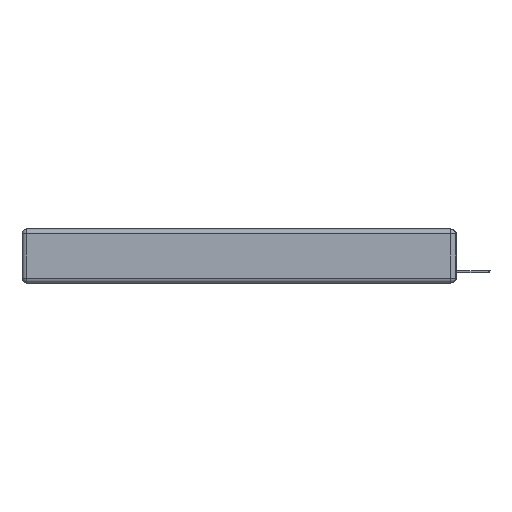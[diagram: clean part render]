
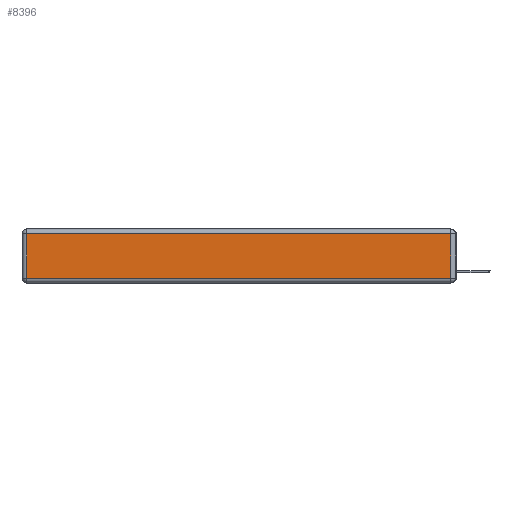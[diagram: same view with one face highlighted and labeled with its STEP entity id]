
A CAD part, left-side view. The second image highlights one B-rep face of the part: STEP entity #8396.
In plain terms, the highlighted planar face has unit normal (-1, 0, 0).
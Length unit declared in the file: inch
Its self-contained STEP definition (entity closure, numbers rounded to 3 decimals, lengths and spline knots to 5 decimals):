
#834 = DIRECTION ( 'NONE',  ( 0., -1., 0. ) ) ;
#1921 = CARTESIAN_POINT ( 'NONE',  ( 0., 0.03, -0.313 ) ) ;
#1926 = VECTOR ( 'NONE', #834, 39.37008 ) ;
#2035 = CARTESIAN_POINT ( 'NONE',  ( 0., 0.03, -0.03 ) ) ;
#2596 = DIRECTION ( 'NONE',  ( -1., 0., 0. ) ) ;
#2621 = ORIENTED_EDGE ( 'NONE', *, *, #5702, .T. ) ;
#3609 = DIRECTION ( 'NONE',  ( 0., 0., 1. ) ) ;
#3985 = VECTOR ( 'NONE', #3609, 39.37008 ) ;
#4456 = LINE ( 'NONE', #26668, #16913 ) ;
#4684 = VERTEX_POINT ( 'NONE', #1921 ) ;
#5519 = VERTEX_POINT ( 'NONE', #24535 ) ;
#5702 = EDGE_CURVE ( 'NONE', #12325, #5519, #23433, .T. ) ;
#5783 = CARTESIAN_POINT ( 'NONE',  ( 0., 0.03, -0.343 ) ) ;
#6226 = DIRECTION ( 'NONE',  ( 0., 1., 0. ) ) ;
#6481 = CARTESIAN_POINT ( 'NONE',  ( 0., 0., -0.313 ) ) ;
#6991 = VERTEX_POINT ( 'NONE', #16761 ) ;
#7860 = EDGE_CURVE ( 'NONE', #6991, #4684, #19782, .T. ) ;
#8375 = EDGE_LOOP ( 'NONE', ( #10088, #24969, #2621, #25903 ) ) ;
#8396 = ADVANCED_FACE ( 'NONE', ( #23601 ), #25797, .T. ) ;
#9207 = DIRECTION ( 'NONE',  ( 0., 0., -1. ) ) ;
#10088 = ORIENTED_EDGE ( 'NONE', *, *, #7860, .T. ) ;
#11227 = VECTOR ( 'NONE', #6226, 39.37008 ) ;
#11928 = LINE ( 'NONE', #5783, #3985 ) ;
#12325 = VERTEX_POINT ( 'NONE', #2035 ) ;
#14876 = EDGE_CURVE ( 'NONE', #5519, #6991, #4456, .T. ) ;
#15117 = DIRECTION ( 'NONE',  ( 0., 0., 1. ) ) ;
#16761 = CARTESIAN_POINT ( 'NONE',  ( 0., 2.72, -0.313 ) ) ;
#16913 = VECTOR ( 'NONE', #9207, 39.37008 ) ;
#19782 = LINE ( 'NONE', #6481, #1926 ) ;
#19796 = AXIS2_PLACEMENT_3D ( 'NONE', #21819, #2596, #15117 ) ;
#21819 = CARTESIAN_POINT ( 'NONE',  ( 0., 0., -0.343 ) ) ;
#22089 = EDGE_CURVE ( 'NONE', #4684, #12325, #11928, .T. ) ;
#23162 = CARTESIAN_POINT ( 'NONE',  ( 0., 2.75, -0.03 ) ) ;
#23433 = LINE ( 'NONE', #23162, #11227 ) ;
#23601 = FACE_OUTER_BOUND ( 'NONE', #8375, .T. ) ;
#24535 = CARTESIAN_POINT ( 'NONE',  ( 0., 2.72, -0.03 ) ) ;
#24969 = ORIENTED_EDGE ( 'NONE', *, *, #22089, .T. ) ;
#25797 = PLANE ( 'NONE',  #19796 ) ;
#25903 = ORIENTED_EDGE ( 'NONE', *, *, #14876, .T. ) ;
#26668 = CARTESIAN_POINT ( 'NONE',  ( 0., 2.72, -0.343 ) ) ;
